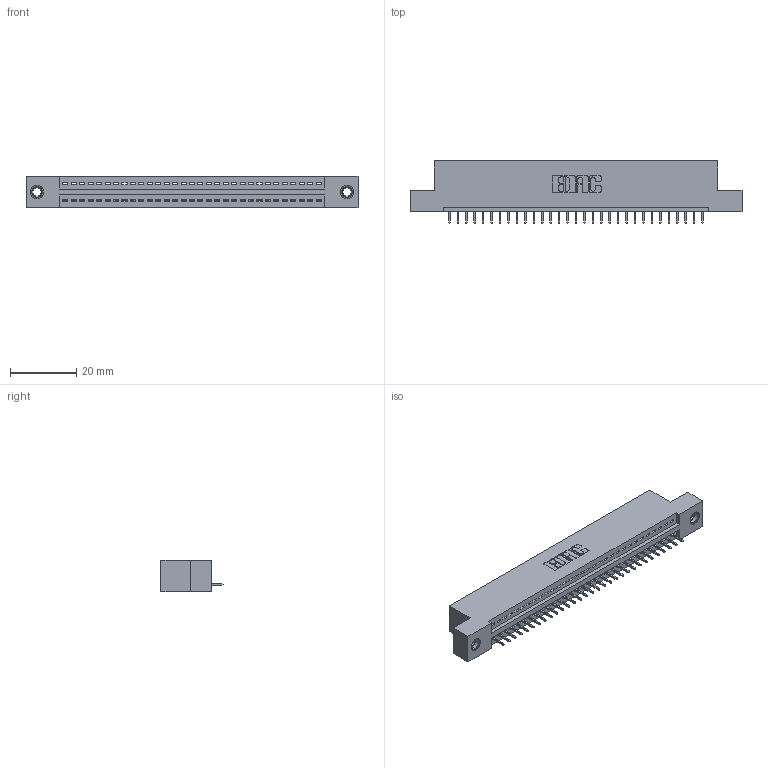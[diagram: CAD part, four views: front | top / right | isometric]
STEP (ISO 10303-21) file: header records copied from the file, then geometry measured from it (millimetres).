
FILE_DESCRIPTION (( 'STEP AP203' ), '1' );
FILE_NAME ('395-031-525-107.STEP', '2020-09-23T20:22:38', ( '' ), ( '' ), 'SwSTEP 2.0', 'SolidWorks 2020', '' );
FILE_SCHEMA (( 'CONFIG_CONTROL_DESIGN' ));
Length unit declared in the file: inch
Products named in the file (4): 345 Part_Flush Mounting Lugs - 0.156 Dia-TI; 345-292-001_345-293-125; 345-250-001_345-250-005-103; 395-031-525-107
Assembly tree (34 placements, depth 2):
  395-031-525-107
    345 Part_Flush Mounting Lugs - 0.156 Dia-TI
    345-292-001_345-293-125  x31
    345-250-001_345-250-005-103  x2
Bounding box: 99.95 x 18.72 x 9.4 mm (x, y, z)
Volume: 9263.1 mm3; surface area: 11770.7 mm2
Topology: 34 solids, 34 shells, 2108 faces, 6057 edges, 3906 vertices
Faces by surface type: plane 1538, cylinder 554, cone 12, torus 4
Entity records: 26072 total; most frequent: CARTESIAN_POINT 4496, ORIENTED_EDGE 4454, DIRECTION 3971, EDGE_CURVE 2227, VECTOR 1955, LINE 1955, VERTEX_POINT 1476, AXIS2_PLACEMENT_3D 1008
